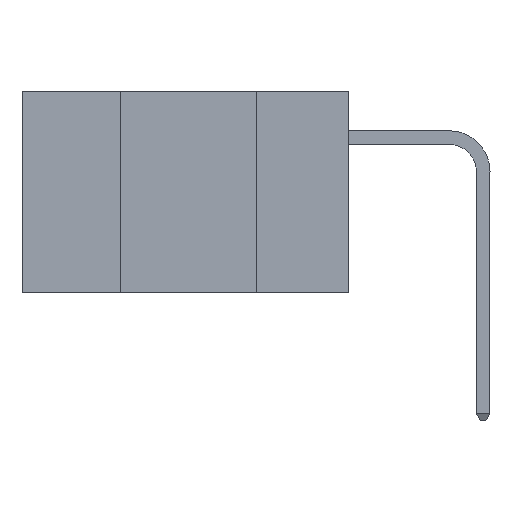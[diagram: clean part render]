
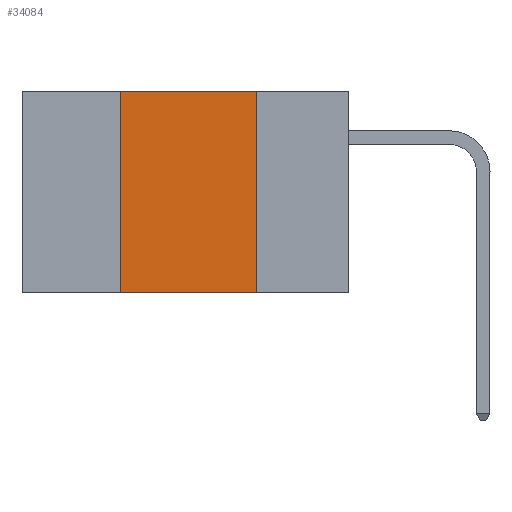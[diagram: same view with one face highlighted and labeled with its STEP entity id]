
A CAD part, left-side view. The second image highlights one B-rep face of the part: STEP entity #34084.
In plain terms, the highlighted planar face has unit normal (-1, 0, 0).
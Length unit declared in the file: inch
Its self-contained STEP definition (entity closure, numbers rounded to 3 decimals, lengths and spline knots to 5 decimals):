
#1282 = EDGE_CURVE ( 'NONE', #18631, #30589, #7615, .T. ) ;
#2218 = VECTOR ( 'NONE', #4629, 39.37008 ) ;
#3173 = DIRECTION ( 'NONE',  ( 0., 0., -1. ) ) ;
#3651 = LINE ( 'NONE', #35526, #32732 ) ;
#3916 = CARTESIAN_POINT ( 'NONE',  ( 0., 0.17, -0.37 ) ) ;
#4232 = VERTEX_POINT ( 'NONE', #29683 ) ;
#4629 = DIRECTION ( 'NONE',  ( 0., -1., 0. ) ) ;
#6254 = ORIENTED_EDGE ( 'NONE', *, *, #18104, .T. ) ;
#6429 = ORIENTED_EDGE ( 'NONE', *, *, #16921, .F. ) ;
#7615 = LINE ( 'NONE', #12815, #35301 ) ;
#8424 = VERTEX_POINT ( 'NONE', #3916 ) ;
#8952 = FACE_OUTER_BOUND ( 'NONE', #20010, .T. ) ;
#9746 = CARTESIAN_POINT ( 'NONE',  ( 0., 0.42, 0. ) ) ;
#12815 = CARTESIAN_POINT ( 'NONE',  ( 0., 0.6, 0. ) ) ;
#13089 = CARTESIAN_POINT ( 'NONE',  ( 0., 0.6, -0.37 ) ) ;
#16281 = EDGE_CURVE ( 'NONE', #4232, #18631, #21963, .T. ) ;
#16921 = EDGE_CURVE ( 'NONE', #30589, #8424, #3651, .T. ) ;
#17370 = PLANE ( 'NONE',  #34583 ) ;
#18104 = EDGE_CURVE ( 'NONE', #4232, #8424, #23954, .T. ) ;
#18405 = ORIENTED_EDGE ( 'NONE', *, *, #1282, .F. ) ;
#18631 = VERTEX_POINT ( 'NONE', #9746 ) ;
#18883 = DIRECTION ( 'NONE',  ( 0., -1., 0. ) ) ;
#18886 = CARTESIAN_POINT ( 'NONE',  ( 0., 0.42, 0. ) ) ;
#20010 = EDGE_LOOP ( 'NONE', ( #6429, #18405, #33187, #6254 ) ) ;
#20242 = DIRECTION ( 'NONE',  ( 1., 0., 0. ) ) ;
#21692 = DIRECTION ( 'NONE',  ( 0., 0., 1. ) ) ;
#21963 = LINE ( 'NONE', #18886, #35779 ) ;
#23954 = LINE ( 'NONE', #13089, #2218 ) ;
#27301 = DIRECTION ( 'NONE',  ( 0., 0., -1. ) ) ;
#29683 = CARTESIAN_POINT ( 'NONE',  ( 0., 0.42, -0.37 ) ) ;
#30589 = VERTEX_POINT ( 'NONE', #34502 ) ;
#32732 = VECTOR ( 'NONE', #27301, 39.37008 ) ;
#33187 = ORIENTED_EDGE ( 'NONE', *, *, #16281, .F. ) ;
#34045 = CARTESIAN_POINT ( 'NONE',  ( 0., 0.6, 0. ) ) ;
#34084 = ADVANCED_FACE ( 'NONE', ( #8952 ), #17370, .F. ) ;
#34502 = CARTESIAN_POINT ( 'NONE',  ( 0., 0.17, 0. ) ) ;
#34583 = AXIS2_PLACEMENT_3D ( 'NONE', #34045, #20242, #3173 ) ;
#35301 = VECTOR ( 'NONE', #18883, 39.37008 ) ;
#35526 = CARTESIAN_POINT ( 'NONE',  ( 0., 0.17, 0. ) ) ;
#35779 = VECTOR ( 'NONE', #21692, 39.37008 ) ;
